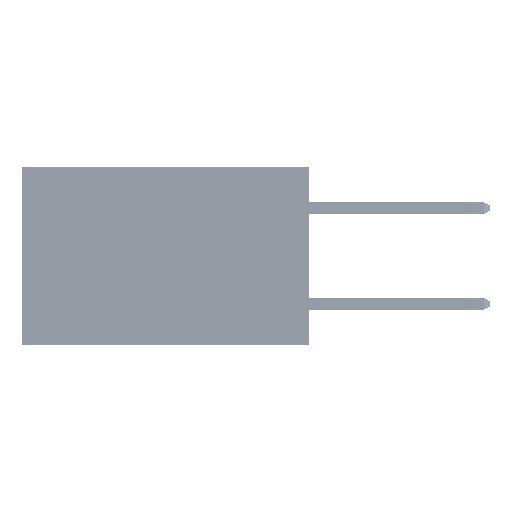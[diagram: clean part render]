
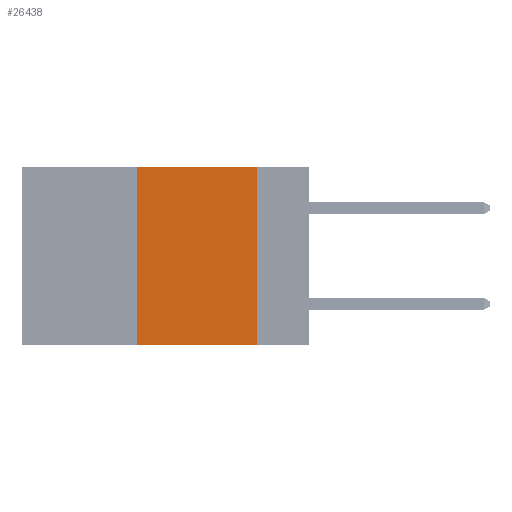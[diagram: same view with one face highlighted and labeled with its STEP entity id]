
A CAD part, left-side view. The second image highlights one B-rep face of the part: STEP entity #26438.
In plain terms, the highlighted planar face has unit normal (-1, 0, 0).
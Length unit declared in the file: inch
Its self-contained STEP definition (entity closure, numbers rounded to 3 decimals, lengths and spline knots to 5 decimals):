
#877 = DIRECTION ( 'NONE',  ( 1., 0., 0. ) ) ;
#1402 = DIRECTION ( 'NONE',  ( 0., 0., -1. ) ) ;
#3232 = DIRECTION ( 'NONE',  ( 0., -1., 0. ) ) ;
#3428 = VECTOR ( 'NONE', #3232, 39.37008 ) ;
#3911 = CARTESIAN_POINT ( 'NONE',  ( 0., 0.6, 0. ) ) ;
#3927 = CARTESIAN_POINT ( 'NONE',  ( 0., 0.36, 0. ) ) ;
#7084 = DIRECTION ( 'NONE',  ( 0., 0., -1. ) ) ;
#7897 = FACE_OUTER_BOUND ( 'NONE', #49624, .T. ) ;
#13395 = CARTESIAN_POINT ( 'NONE',  ( 0., 0.11, -0.37 ) ) ;
#15340 = DIRECTION ( 'NONE',  ( 0., 0., 1. ) ) ;
#17858 = LINE ( 'NONE', #3911, #3428 ) ;
#17992 = EDGE_CURVE ( 'NONE', #30056, #47269, #17858, .T. ) ;
#18836 = CARTESIAN_POINT ( 'NONE',  ( 0., 0.11, 0. ) ) ;
#21823 = LINE ( 'NONE', #3927, #23074 ) ;
#23074 = VECTOR ( 'NONE', #15340, 39.37008 ) ;
#24724 = CARTESIAN_POINT ( 'NONE',  ( 0., 0.36, 0. ) ) ;
#25385 = PLANE ( 'NONE',  #44607 ) ;
#26117 = EDGE_CURVE ( 'NONE', #42067, #41569, #45648, .T. ) ;
#26438 = ADVANCED_FACE ( 'NONE', ( #7897 ), #25385, .F. ) ;
#26928 = ORIENTED_EDGE ( 'NONE', *, *, #40076, .F. ) ;
#29022 = ORIENTED_EDGE ( 'NONE', *, *, #26117, .T. ) ;
#30056 = VERTEX_POINT ( 'NONE', #24724 ) ;
#31298 = CARTESIAN_POINT ( 'NONE',  ( 0., 0.6, -0.37 ) ) ;
#34078 = EDGE_CURVE ( 'NONE', #47269, #41569, #44844, .T. ) ;
#36129 = VECTOR ( 'NONE', #43739, 39.37008 ) ;
#40076 = EDGE_CURVE ( 'NONE', #42067, #30056, #21823, .T. ) ;
#40821 = CARTESIAN_POINT ( 'NONE',  ( 0., 0.6, 0. ) ) ;
#41569 = VERTEX_POINT ( 'NONE', #13395 ) ;
#41899 = CARTESIAN_POINT ( 'NONE',  ( 0., 0.36, -0.37 ) ) ;
#42067 = VERTEX_POINT ( 'NONE', #41899 ) ;
#43564 = VECTOR ( 'NONE', #7084, 39.37008 ) ;
#43739 = DIRECTION ( 'NONE',  ( 0., -1., 0. ) ) ;
#44607 = AXIS2_PLACEMENT_3D ( 'NONE', #40821, #877, #1402 ) ;
#44844 = LINE ( 'NONE', #18836, #43564 ) ;
#45648 = LINE ( 'NONE', #31298, #36129 ) ;
#45814 = ORIENTED_EDGE ( 'NONE', *, *, #34078, .F. ) ;
#46168 = CARTESIAN_POINT ( 'NONE',  ( 0., 0.11, 0. ) ) ;
#47269 = VERTEX_POINT ( 'NONE', #46168 ) ;
#48734 = ORIENTED_EDGE ( 'NONE', *, *, #17992, .F. ) ;
#49624 = EDGE_LOOP ( 'NONE', ( #45814, #48734, #26928, #29022 ) ) ;
